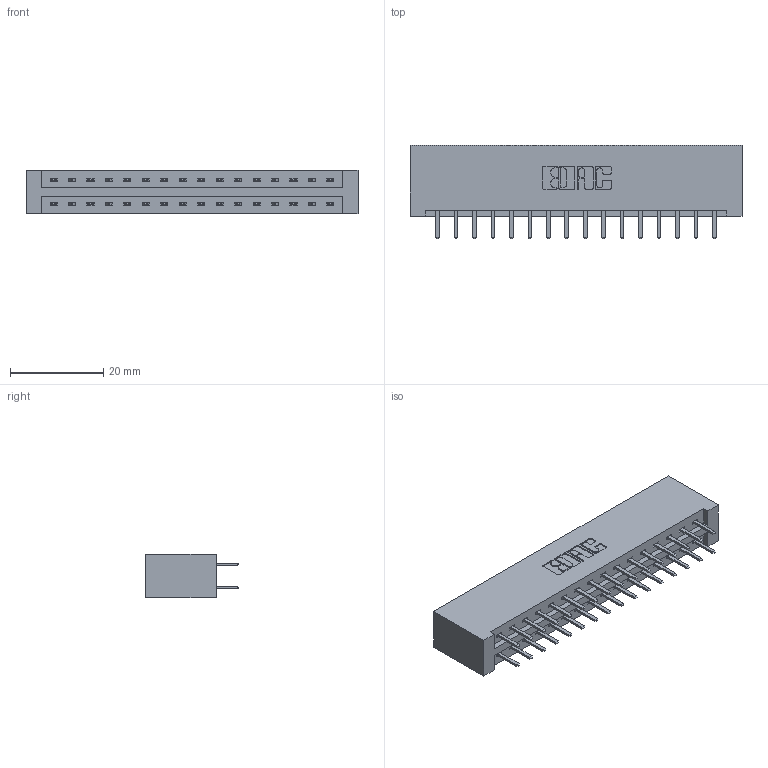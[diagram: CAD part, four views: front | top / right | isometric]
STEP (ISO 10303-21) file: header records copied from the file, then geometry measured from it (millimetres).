
FILE_DESCRIPTION (( 'STEP AP203' ), '1' );
FILE_NAME ('337-032-520-201.STEP', '2019-10-08T19:09:24', ( '' ), ( '' ), 'SwSTEP 2.0', 'SolidWorks 2016', '' );
FILE_SCHEMA (( 'CONFIG_CONTROL_DESIGN' ));
Length unit declared in the file: inch
Products named in the file (3): 337-032-520-201; 345-292-001_345-293-120; 337 Part_No Mounting Lugs
Assembly tree (33 placements, depth 2):
  337-032-520-201
    337 Part_No Mounting Lugs
    345-292-001_345-293-120  x32
Bounding box: 71.27 x 20.02 x 9.4 mm (x, y, z)
Volume: 7911.8 mm3; surface area: 8707.8 mm2
Topology: 33 solids, 33 shells, 1962 faces, 5695 edges, 3710 vertices
Faces by surface type: plane 1346, cylinder 616
Entity records: 15605 total; most frequent: CARTESIAN_POINT 2662, ORIENTED_EDGE 2586, DIRECTION 2293, EDGE_CURVE 1293, LINE 1169, VECTOR 1169, VERTEX_POINT 858, AXIS2_PLACEMENT_3D 562
